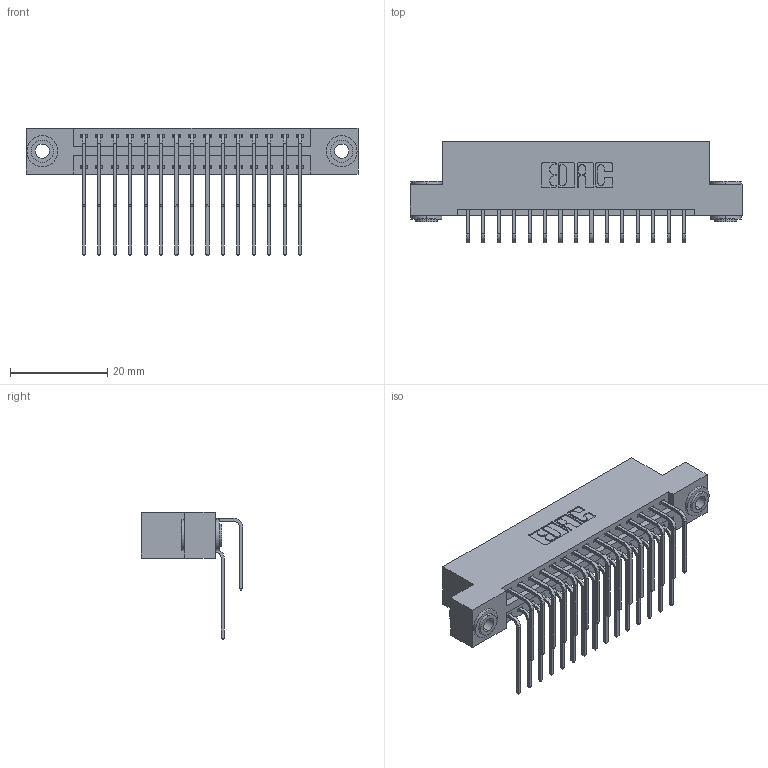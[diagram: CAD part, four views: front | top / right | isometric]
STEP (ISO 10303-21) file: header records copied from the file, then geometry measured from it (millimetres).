
FILE_DESCRIPTION (( 'STEP AP203' ), '1' );
FILE_NAME ('346-030-559-203.STEP', '2022-05-19T17:05:23', ( '' ), ( '' ), 'SwSTEP 2.0', 'SolidWorks 2020', '' );
FILE_SCHEMA (( 'CONFIG_CONTROL_DESIGN' ));
Length unit declared in the file: inch
Products named in the file (5): 346 Part_Flush Mounting Lugs - 0.156 Dia-TH; 346-030-559-203; 345-292-001_558 559 Tail - 1; 345-250-002_345-250-002-102; 345-292-001_559 Tail - 2
Assembly tree (33 placements, depth 2):
  346-030-559-203
    346 Part_Flush Mounting Lugs - 0.156 Dia-TH
    345-292-001_558 559 Tail - 1  x15
    345-292-001_559 Tail - 2  x15
    345-250-002_345-250-002-102  x2
Bounding box: 68.2 x 20.89 x 26.16 mm (x, y, z)
Volume: 6614.9 mm3; surface area: 9747.2 mm2
Topology: 33 solids, 33 shells, 1794 faces, 5271 edges, 3470 vertices
Faces by surface type: plane 1210, cylinder 576, cone 8
Entity records: 16274 total; most frequent: CARTESIAN_POINT 2752, ORIENTED_EDGE 2626, DIRECTION 2479, EDGE_CURVE 1313, LINE 1057, VECTOR 1057, VERTEX_POINT 870, AXIS2_PLACEMENT_3D 711
